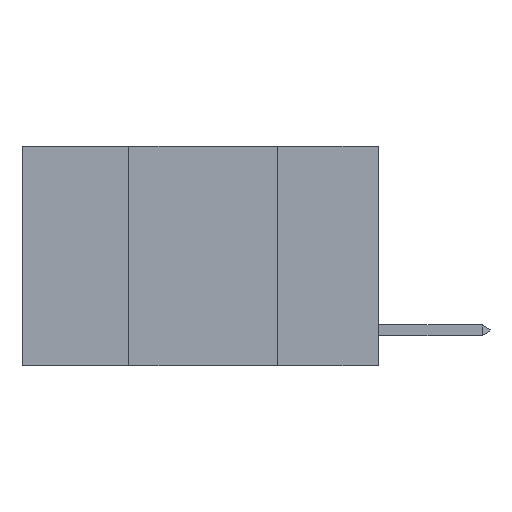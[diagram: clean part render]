
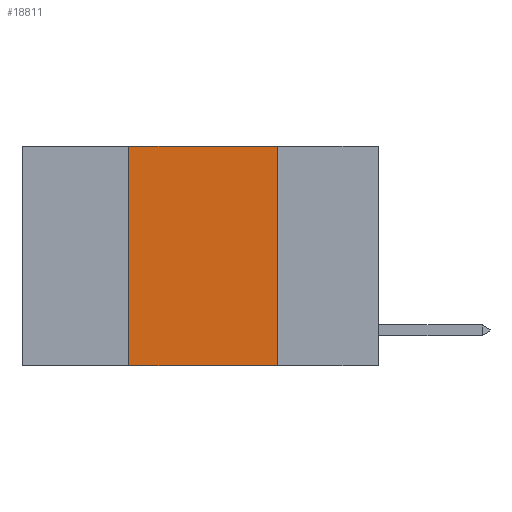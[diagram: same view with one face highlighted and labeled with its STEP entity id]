
A CAD part, left-side view. The second image highlights one B-rep face of the part: STEP entity #18811.
In plain terms, the highlighted planar face has unit normal (-1, 0, 0).
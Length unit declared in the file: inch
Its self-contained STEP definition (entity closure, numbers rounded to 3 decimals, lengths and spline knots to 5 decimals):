
#91 = VERTEX_POINT ( 'NONE', #4406 ) ;
#202 = VERTEX_POINT ( 'NONE', #23472 ) ;
#291 = DIRECTION ( 'NONE',  ( 0., 0., -1. ) ) ;
#1194 = ORIENTED_EDGE ( 'NONE', *, *, #4723, .T. ) ;
#1346 = LINE ( 'NONE', #23669, #20048 ) ;
#1909 = CARTESIAN_POINT ( 'NONE',  ( 0., 0.42, 0. ) ) ;
#3149 = DIRECTION ( 'NONE',  ( 1., 0., 0. ) ) ;
#3427 = ORIENTED_EDGE ( 'NONE', *, *, #29672, .F. ) ;
#4406 = CARTESIAN_POINT ( 'NONE',  ( 0., 0.17, 0. ) ) ;
#4723 = EDGE_CURVE ( 'NONE', #15892, #202, #10934, .T. ) ;
#5710 = AXIS2_PLACEMENT_3D ( 'NONE', #7640, #3149, #19536 ) ;
#7320 = CARTESIAN_POINT ( 'NONE',  ( 0., 0.42, -0.37 ) ) ;
#7640 = CARTESIAN_POINT ( 'NONE',  ( 0., 0.6, 0. ) ) ;
#8169 = ORIENTED_EDGE ( 'NONE', *, *, #29761, .F. ) ;
#8871 = VERTEX_POINT ( 'NONE', #1909 ) ;
#9675 = DIRECTION ( 'NONE',  ( 0., -1., 0. ) ) ;
#10416 = VECTOR ( 'NONE', #291, 39.37008 ) ;
#10934 = LINE ( 'NONE', #29539, #21928 ) ;
#11296 = FACE_OUTER_BOUND ( 'NONE', #21811, .T. ) ;
#12346 = CARTESIAN_POINT ( 'NONE',  ( 0., 0.42, 0. ) ) ;
#12430 = PLANE ( 'NONE',  #5710 ) ;
#15884 = EDGE_CURVE ( 'NONE', #8871, #91, #1346, .T. ) ;
#15892 = VERTEX_POINT ( 'NONE', #7320 ) ;
#18811 = ADVANCED_FACE ( 'NONE', ( #11296 ), #12430, .F. ) ;
#19536 = DIRECTION ( 'NONE',  ( 0., 0., -1. ) ) ;
#20048 = VECTOR ( 'NONE', #9675, 39.37008 ) ;
#20627 = ORIENTED_EDGE ( 'NONE', *, *, #15884, .F. ) ;
#21811 = EDGE_LOOP ( 'NONE', ( #3427, #20627, #8169, #1194 ) ) ;
#21928 = VECTOR ( 'NONE', #24900, 39.37008 ) ;
#23472 = CARTESIAN_POINT ( 'NONE',  ( 0., 0.17, -0.37 ) ) ;
#23496 = CARTESIAN_POINT ( 'NONE',  ( 0., 0.17, 0. ) ) ;
#23669 = CARTESIAN_POINT ( 'NONE',  ( 0., 0.6, 0. ) ) ;
#24900 = DIRECTION ( 'NONE',  ( 0., -1., 0. ) ) ;
#25383 = VECTOR ( 'NONE', #28645, 39.37008 ) ;
#26133 = LINE ( 'NONE', #12346, #25383 ) ;
#28645 = DIRECTION ( 'NONE',  ( 0., 0., 1. ) ) ;
#29027 = LINE ( 'NONE', #23496, #10416 ) ;
#29539 = CARTESIAN_POINT ( 'NONE',  ( 0., 0.6, -0.37 ) ) ;
#29672 = EDGE_CURVE ( 'NONE', #91, #202, #29027, .T. ) ;
#29761 = EDGE_CURVE ( 'NONE', #15892, #8871, #26133, .T. ) ;
